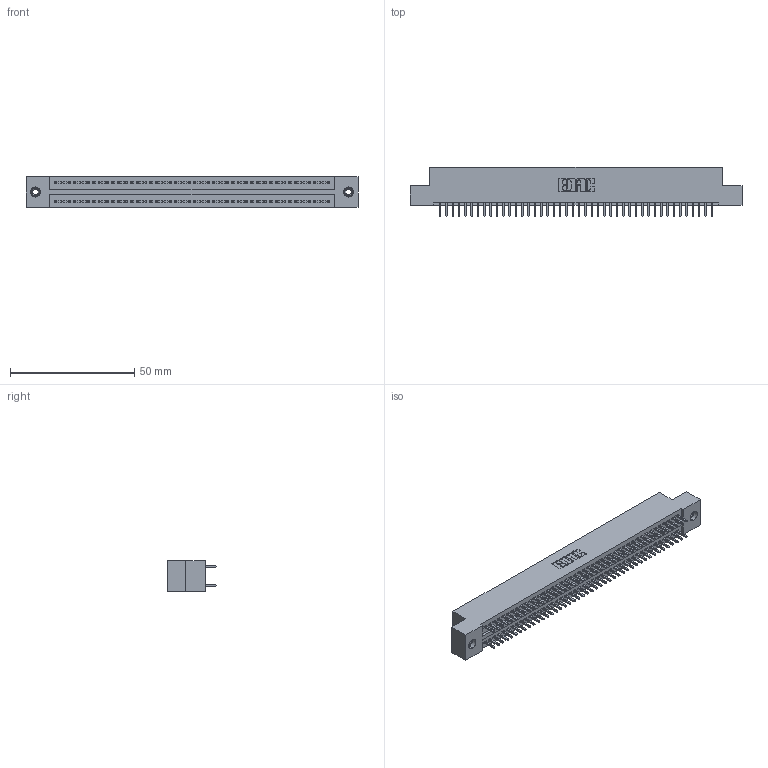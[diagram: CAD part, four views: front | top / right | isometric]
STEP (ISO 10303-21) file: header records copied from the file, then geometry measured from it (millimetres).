
FILE_DESCRIPTION (( 'STEP AP203' ), '1' );
FILE_NAME ('325-088-520-208.STEP', '2020-02-25T05:26:43', ( '' ), ( '' ), 'SwSTEP 2.0', 'SolidWorks 2016', '' );
FILE_SCHEMA (( 'CONFIG_CONTROL_DESIGN' ));
Length unit declared in the file: inch
Products named in the file (4): 325 Part_TI; 345-250-001_345-250-003-102; 325-088-520-208; 325-292-001_325-293-120
Assembly tree (91 placements, depth 2):
  325-088-520-208
    325 Part_TI
    325-292-001_325-293-120  x88
    345-250-001_345-250-003-102  x2
Bounding box: 133.48 x 19.68 x 12.45 mm (x, y, z)
Volume: 17229.5 mm3; surface area: 20737.3 mm2
Topology: 91 solids, 91 shells, 4750 faces, 14087 edges, 9266 vertices
Faces by surface type: plane 3270, cylinder 1464, cone 12, torus 4
Entity records: 29252 total; most frequent: CARTESIAN_POINT 4829, ORIENTED_EDGE 4758, DIRECTION 4153, EDGE_CURVE 2379, LINE 2231, VECTOR 2231, VERTEX_POINT 1580, AXIS2_PLACEMENT_3D 961
